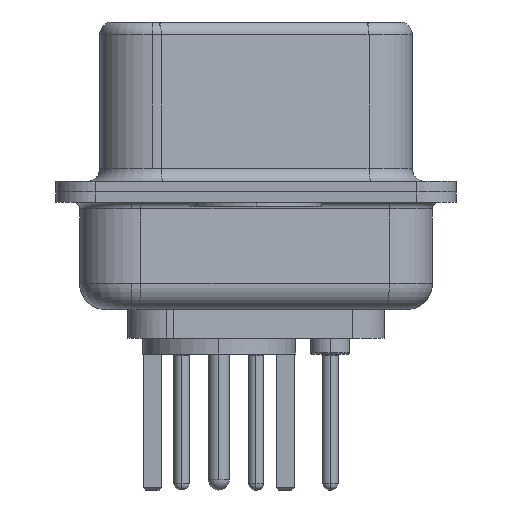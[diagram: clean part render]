
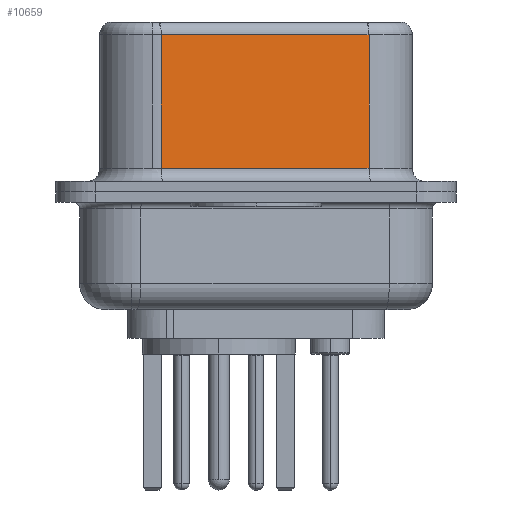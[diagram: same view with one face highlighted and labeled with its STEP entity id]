
A CAD part, left-side view. The second image highlights one B-rep face of the part: STEP entity #10659.
In plain terms, the highlighted planar face has unit normal (-0.985, -0.174, 0).
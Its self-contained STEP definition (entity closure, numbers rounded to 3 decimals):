
#23 = VERTEX_POINT ( 'NONE', #1942 ) ;
#1942 = CARTESIAN_POINT ( 'NONE',  ( 5.132, -4.322, 0.9 ) ) ;
#2940 = CARTESIAN_POINT ( 'NONE',  ( 3.73, 3.628, 6.02 ) ) ;
#3627 = LINE ( 'NONE', #15817, #13468 ) ;
#4967 = DIRECTION ( 'NONE',  ( -0.174, 0.985, 0. ) ) ;
#6115 = DIRECTION ( 'NONE',  ( 0.174, -0.985, 0. ) ) ;
#6984 = EDGE_LOOP ( 'NONE', ( #10199, #22395, #24504, #9532 ) ) ;
#8122 = VECTOR ( 'NONE', #9224, 1000. ) ;
#8437 = VECTOR ( 'NONE', #13669, 1000. ) ;
#9080 = LINE ( 'NONE', #24032, #8437 ) ;
#9224 = DIRECTION ( 'NONE',  ( -0.174, 0.985, 0. ) ) ;
#9532 = ORIENTED_EDGE ( 'NONE', *, *, #25007, .T. ) ;
#10199 = ORIENTED_EDGE ( 'NONE', *, *, #12496, .F. ) ;
#10659 = ADVANCED_FACE ( 'NONE', ( #19914 ), #13304, .F. ) ;
#11096 = VERTEX_POINT ( 'NONE', #21152 ) ;
#12496 = EDGE_CURVE ( 'NONE', #20089, #23, #9080, .T. ) ;
#13304 = PLANE ( 'NONE',  #22995 ) ;
#13468 = VECTOR ( 'NONE', #17953, 1000. ) ;
#13524 = CARTESIAN_POINT ( 'NONE',  ( 5.132, -4.322, 6.02 ) ) ;
#13669 = DIRECTION ( 'NONE',  ( 0., 0., -1. ) ) ;
#13698 = LINE ( 'NONE', #21699, #8122 ) ;
#15817 = CARTESIAN_POINT ( 'NONE',  ( 3.73, 3.628, 6.52 ) ) ;
#17516 = DIRECTION ( 'NONE',  ( 0.985, 0.174, 0. ) ) ;
#17953 = DIRECTION ( 'NONE',  ( 0., 0., -1. ) ) ;
#19326 = EDGE_CURVE ( 'NONE', #20089, #24018, #13698, .T. ) ;
#19366 = VECTOR ( 'NONE', #6115, 1000. ) ;
#19914 = FACE_OUTER_BOUND ( 'NONE', #6984, .T. ) ;
#20089 = VERTEX_POINT ( 'NONE', #13524 ) ;
#20767 = CARTESIAN_POINT ( 'NONE',  ( 5.132, -4.322, 0.9 ) ) ;
#21152 = CARTESIAN_POINT ( 'NONE',  ( 3.73, 3.628, 0.9 ) ) ;
#21699 = CARTESIAN_POINT ( 'NONE',  ( 5.132, -4.322, 6.02 ) ) ;
#22395 = ORIENTED_EDGE ( 'NONE', *, *, #19326, .T. ) ;
#22995 = AXIS2_PLACEMENT_3D ( 'NONE', #23676, #17516, #4967 ) ;
#23676 = CARTESIAN_POINT ( 'NONE',  ( 5.132, -4.322, 6.52 ) ) ;
#24018 = VERTEX_POINT ( 'NONE', #2940 ) ;
#24032 = CARTESIAN_POINT ( 'NONE',  ( 5.132, -4.322, 6.52 ) ) ;
#24504 = ORIENTED_EDGE ( 'NONE', *, *, #24773, .T. ) ;
#24773 = EDGE_CURVE ( 'NONE', #24018, #11096, #3627, .T. ) ;
#25007 = EDGE_CURVE ( 'NONE', #11096, #23, #25454, .T. ) ;
#25454 = LINE ( 'NONE', #20767, #19366 ) ;
